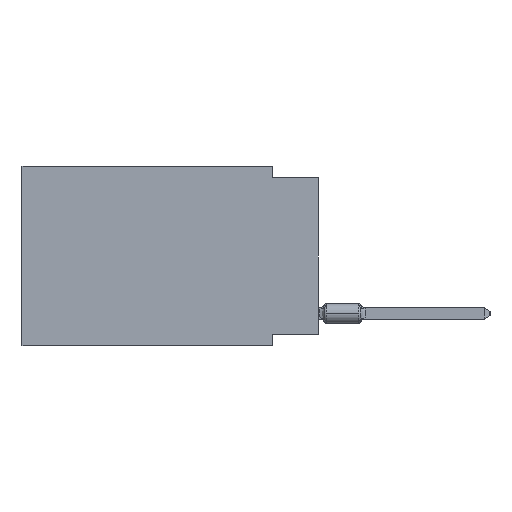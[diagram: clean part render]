
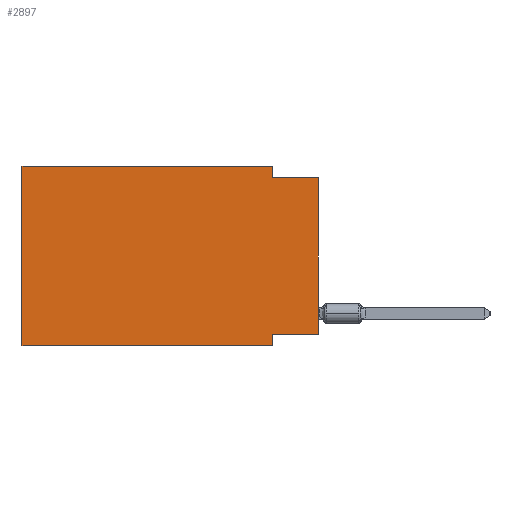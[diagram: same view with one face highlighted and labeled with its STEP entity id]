
A CAD part, left-side view. The second image highlights one B-rep face of the part: STEP entity #2897.
In plain terms, the highlighted planar face has unit normal (-1, 0, 0).
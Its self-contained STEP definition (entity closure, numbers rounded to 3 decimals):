
#885 = DIRECTION ( 'NONE',  ( 0., 0., 1. ) ) ;
#1302 = VERTEX_POINT ( 'NONE', #6913 ) ;
#1486 = EDGE_CURVE ( 'NONE', #13713, #55541, #36085, .T. ) ;
#2090 = EDGE_CURVE ( 'NONE', #1302, #27897, #35860, .T. ) ;
#2897 = ADVANCED_FACE ( 'NONE', ( #21099 ), #12317, .F. ) ;
#4072 = DIRECTION ( 'NONE',  ( 0., -1., 0. ) ) ;
#6913 = CARTESIAN_POINT ( 'NONE',  ( 0., 16.383, -9.906 ) ) ;
#7032 = CARTESIAN_POINT ( 'NONE',  ( 0., 0., -0.635 ) ) ;
#7097 = CARTESIAN_POINT ( 'NONE',  ( 0., 0., -9.271 ) ) ;
#8206 = LINE ( 'NONE', #53611, #8662 ) ;
#8662 = VECTOR ( 'NONE', #4072, 1000. ) ;
#10117 = EDGE_LOOP ( 'NONE', ( #50927, #44477, #31518, #15968, #26084, #45718, #17340, #34519 ) ) ;
#11022 = AXIS2_PLACEMENT_3D ( 'NONE', #44242, #43672, #29901 ) ;
#12317 = PLANE ( 'NONE',  #11022 ) ;
#12660 = VECTOR ( 'NONE', #13594, 1000. ) ;
#13126 = DIRECTION ( 'NONE',  ( 0., -1., 0. ) ) ;
#13594 = DIRECTION ( 'NONE',  ( 0., 0., 1. ) ) ;
#13713 = VERTEX_POINT ( 'NONE', #38659 ) ;
#13826 = DIRECTION ( 'NONE',  ( 0., 0., -1. ) ) ;
#14101 = LINE ( 'NONE', #31962, #51555 ) ;
#15215 = EDGE_CURVE ( 'NONE', #50011, #35254, #14101, .T. ) ;
#15469 = VECTOR ( 'NONE', #26064, 1000. ) ;
#15968 = ORIENTED_EDGE ( 'NONE', *, *, #37746, .F. ) ;
#16611 = EDGE_CURVE ( 'NONE', #1302, #55541, #8206, .T. ) ;
#17340 = ORIENTED_EDGE ( 'NONE', *, *, #1486, .F. ) ;
#17973 = CARTESIAN_POINT ( 'NONE',  ( 0., 0., -9.271 ) ) ;
#20013 = LINE ( 'NONE', #55773, #41060 ) ;
#21099 = FACE_OUTER_BOUND ( 'NONE', #10117, .T. ) ;
#22191 = LINE ( 'NONE', #30411, #43845 ) ;
#26064 = DIRECTION ( 'NONE',  ( 0., 0., -1. ) ) ;
#26084 = ORIENTED_EDGE ( 'NONE', *, *, #2090, .F. ) ;
#27562 = EDGE_CURVE ( 'NONE', #50011, #13713, #39317, .T. ) ;
#27897 = VERTEX_POINT ( 'NONE', #42487 ) ;
#27918 = CARTESIAN_POINT ( 'NONE',  ( 0., 2.54, 0. ) ) ;
#29090 = DIRECTION ( 'NONE',  ( 0., -1., 0. ) ) ;
#29901 = DIRECTION ( 'NONE',  ( 0., 0., -1. ) ) ;
#30081 = CARTESIAN_POINT ( 'NONE',  ( 0., 2.54, -0.635 ) ) ;
#30411 = CARTESIAN_POINT ( 'NONE',  ( 0., 16.383, 0. ) ) ;
#30986 = VECTOR ( 'NONE', #39028, 1000. ) ;
#31518 = ORIENTED_EDGE ( 'NONE', *, *, #41415, .F. ) ;
#31962 = CARTESIAN_POINT ( 'NONE',  ( 0., 0., 0. ) ) ;
#34467 = CARTESIAN_POINT ( 'NONE',  ( 0., 2.54, -9.906 ) ) ;
#34519 = ORIENTED_EDGE ( 'NONE', *, *, #27562, .F. ) ;
#34815 = VERTEX_POINT ( 'NONE', #27918 ) ;
#35210 = VECTOR ( 'NONE', #13826, 1000. ) ;
#35254 = VERTEX_POINT ( 'NONE', #7032 ) ;
#35860 = LINE ( 'NONE', #53747, #12660 ) ;
#36085 = LINE ( 'NONE', #53977, #35210 ) ;
#37746 = EDGE_CURVE ( 'NONE', #27897, #34815, #22191, .T. ) ;
#38659 = CARTESIAN_POINT ( 'NONE',  ( 0., 2.54, -9.271 ) ) ;
#39028 = DIRECTION ( 'NONE',  ( 0., 1., 0. ) ) ;
#39317 = LINE ( 'NONE', #7097, #30986 ) ;
#41060 = VECTOR ( 'NONE', #29090, 1000. ) ;
#41415 = EDGE_CURVE ( 'NONE', #34815, #49514, #43680, .T. ) ;
#42487 = CARTESIAN_POINT ( 'NONE',  ( 0., 16.383, 0. ) ) ;
#43672 = DIRECTION ( 'NONE',  ( 1., 0., 0. ) ) ;
#43680 = LINE ( 'NONE', #48356, #15469 ) ;
#43845 = VECTOR ( 'NONE', #13126, 1000. ) ;
#44242 = CARTESIAN_POINT ( 'NONE',  ( 0., 16.383, 0. ) ) ;
#44477 = ORIENTED_EDGE ( 'NONE', *, *, #52384, .F. ) ;
#45718 = ORIENTED_EDGE ( 'NONE', *, *, #16611, .T. ) ;
#48356 = CARTESIAN_POINT ( 'NONE',  ( 0., 2.54, 0. ) ) ;
#49514 = VERTEX_POINT ( 'NONE', #30081 ) ;
#50011 = VERTEX_POINT ( 'NONE', #17973 ) ;
#50927 = ORIENTED_EDGE ( 'NONE', *, *, #15215, .T. ) ;
#51555 = VECTOR ( 'NONE', #885, 1000. ) ;
#52384 = EDGE_CURVE ( 'NONE', #49514, #35254, #20013, .T. ) ;
#53611 = CARTESIAN_POINT ( 'NONE',  ( 0., 16.383, -9.906 ) ) ;
#53747 = CARTESIAN_POINT ( 'NONE',  ( 0., 16.383, 0. ) ) ;
#53977 = CARTESIAN_POINT ( 'NONE',  ( 0., 2.54, -9.906 ) ) ;
#55541 = VERTEX_POINT ( 'NONE', #34467 ) ;
#55773 = CARTESIAN_POINT ( 'NONE',  ( 0., 0., -0.635 ) ) ;
